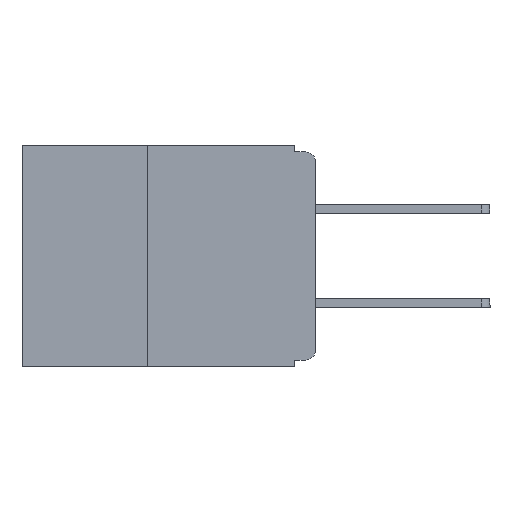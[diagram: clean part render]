
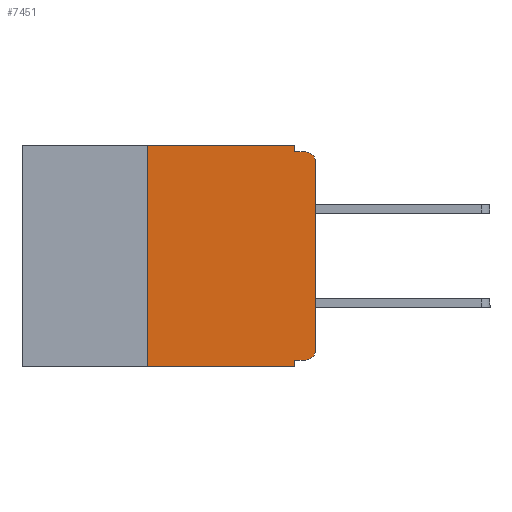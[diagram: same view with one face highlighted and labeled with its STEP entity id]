
A CAD part, left-side view. The second image highlights one B-rep face of the part: STEP entity #7451.
In plain terms, the highlighted planar face has unit normal (-1, 0, 0).
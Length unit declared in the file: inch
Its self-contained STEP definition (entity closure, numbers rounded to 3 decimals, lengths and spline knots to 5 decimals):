
#254 = LINE ( 'NONE', #30132, #18545 ) ;
#297 = CARTESIAN_POINT ( 'NONE',  ( 0., 0.015, -0.01 ) ) ;
#335 = ORIENTED_EDGE ( 'NONE', *, *, #7287, .T. ) ;
#672 = DIRECTION ( 'NONE',  ( 0., -1., 0. ) ) ;
#1065 = VECTOR ( 'NONE', #12411, 39.37008 ) ;
#1700 = CARTESIAN_POINT ( 'NONE',  ( 0., 0., 0. ) ) ;
#1806 = EDGE_LOOP ( 'NONE', ( #30717, #335, #18249, #26218, #25483, #6703, #31536, #11788, #13303, #30813 ) ) ;
#2126 = DIRECTION ( 'NONE',  ( 0., -1., 0. ) ) ;
#2202 = VERTEX_POINT ( 'NONE', #297 ) ;
#2944 = LINE ( 'NONE', #21747, #27592 ) ;
#3209 = CARTESIAN_POINT ( 'NONE',  ( 0., 0.015, -0.305 ) ) ;
#3772 = CARTESIAN_POINT ( 'NONE',  ( 0., 0.25, -0.33 ) ) ;
#4132 = VECTOR ( 'NONE', #2126, 39.37008 ) ;
#4405 = LINE ( 'NONE', #1700, #22552 ) ;
#4862 = DIRECTION ( 'NONE',  ( 0., 0., -1. ) ) ;
#4870 = DIRECTION ( 'NONE',  ( 1., 0., 0. ) ) ;
#4980 = PLANE ( 'NONE',  #14857 ) ;
#5081 = CARTESIAN_POINT ( 'NONE',  ( 0., 0.437, 0. ) ) ;
#5766 = DIRECTION ( 'NONE',  ( 0., 0., -1. ) ) ;
#6234 = VERTEX_POINT ( 'NONE', #24008 ) ;
#6649 = VERTEX_POINT ( 'NONE', #18091 ) ;
#6653 = CARTESIAN_POINT ( 'NONE',  ( 0., 0.25, 0. ) ) ;
#6703 = ORIENTED_EDGE ( 'NONE', *, *, #12889, .F. ) ;
#7101 = CARTESIAN_POINT ( 'NONE',  ( 0., 0.437, 0. ) ) ;
#7257 = VERTEX_POINT ( 'NONE', #7839 ) ;
#7287 = EDGE_CURVE ( 'NONE', #26455, #2202, #21503, .T. ) ;
#7451 = ADVANCED_FACE ( 'NONE', ( #22644 ), #4980, .F. ) ;
#7493 = DIRECTION ( 'NONE',  ( 0., 0., -1. ) ) ;
#7524 = DIRECTION ( 'NONE',  ( -1., 0., 0. ) ) ;
#7559 = CARTESIAN_POINT ( 'NONE',  ( 0., 0.015, -0.025 ) ) ;
#7839 = CARTESIAN_POINT ( 'NONE',  ( 0., 0.015, -0.32 ) ) ;
#10695 = DIRECTION ( 'NONE',  ( 0., -1., 0. ) ) ;
#11396 = CARTESIAN_POINT ( 'NONE',  ( 0., 0.031, 0. ) ) ;
#11788 = ORIENTED_EDGE ( 'NONE', *, *, #17528, .F. ) ;
#11911 = EDGE_CURVE ( 'NONE', #25136, #6649, #254, .T. ) ;
#12411 = DIRECTION ( 'NONE',  ( 0., 0., -1. ) ) ;
#12565 = CIRCLE ( 'NONE', #22914, 0.015 ) ;
#12889 = EDGE_CURVE ( 'NONE', #25136, #25389, #2944, .T. ) ;
#13303 = ORIENTED_EDGE ( 'NONE', *, *, #20411, .F. ) ;
#14413 = VECTOR ( 'NONE', #18692, 39.37008 ) ;
#14503 = VECTOR ( 'NONE', #21837, 39.37008 ) ;
#14857 = AXIS2_PLACEMENT_3D ( 'NONE', #5081, #4870, #4862 ) ;
#16681 = EDGE_CURVE ( 'NONE', #18161, #6234, #21692, .T. ) ;
#17235 = VERTEX_POINT ( 'NONE', #25765 ) ;
#17528 = EDGE_CURVE ( 'NONE', #17235, #6649, #27336, .T. ) ;
#18091 = CARTESIAN_POINT ( 'NONE',  ( 0., 0.031, -0.33 ) ) ;
#18148 = CARTESIAN_POINT ( 'NONE',  ( 0., 0., -0.025 ) ) ;
#18161 = VERTEX_POINT ( 'NONE', #24557 ) ;
#18249 = ORIENTED_EDGE ( 'NONE', *, *, #26424, .F. ) ;
#18545 = VECTOR ( 'NONE', #672, 39.37008 ) ;
#18692 = DIRECTION ( 'NONE',  ( 0., 0., -1. ) ) ;
#20351 = EDGE_CURVE ( 'NONE', #31775, #26455, #4405, .T. ) ;
#20411 = EDGE_CURVE ( 'NONE', #7257, #17235, #21031, .T. ) ;
#20563 = DIRECTION ( 'NONE',  ( -1., 0., 0. ) ) ;
#20694 = EDGE_CURVE ( 'NONE', #7257, #31775, #12565, .T. ) ;
#21031 = LINE ( 'NONE', #29031, #14503 ) ;
#21503 = CIRCLE ( 'NONE', #26906, 0.015 ) ;
#21692 = LINE ( 'NONE', #11396, #14413 ) ;
#21747 = CARTESIAN_POINT ( 'NONE',  ( 0., 0.25, -0.33 ) ) ;
#21837 = DIRECTION ( 'NONE',  ( 0., 1., 0. ) ) ;
#22552 = VECTOR ( 'NONE', #23847, 39.37008 ) ;
#22644 = FACE_OUTER_BOUND ( 'NONE', #1806, .T. ) ;
#22914 = AXIS2_PLACEMENT_3D ( 'NONE', #3209, #20563, #5766 ) ;
#22923 = CARTESIAN_POINT ( 'NONE',  ( 0., 0., -0.01 ) ) ;
#23847 = DIRECTION ( 'NONE',  ( 0., 0., 1. ) ) ;
#24008 = CARTESIAN_POINT ( 'NONE',  ( 0., 0.031, -0.01 ) ) ;
#24183 = DIRECTION ( 'NONE',  ( 0., 0., 1. ) ) ;
#24557 = CARTESIAN_POINT ( 'NONE',  ( 0., 0.031, 0. ) ) ;
#25136 = VERTEX_POINT ( 'NONE', #3772 ) ;
#25389 = VERTEX_POINT ( 'NONE', #6653 ) ;
#25483 = ORIENTED_EDGE ( 'NONE', *, *, #28605, .F. ) ;
#25765 = CARTESIAN_POINT ( 'NONE',  ( 0., 0.031, -0.32 ) ) ;
#26218 = ORIENTED_EDGE ( 'NONE', *, *, #16681, .F. ) ;
#26288 = CARTESIAN_POINT ( 'NONE',  ( 0., 0., -0.305 ) ) ;
#26424 = EDGE_CURVE ( 'NONE', #6234, #2202, #31466, .T. ) ;
#26455 = VERTEX_POINT ( 'NONE', #18148 ) ;
#26906 = AXIS2_PLACEMENT_3D ( 'NONE', #7559, #7524, #7493 ) ;
#27336 = LINE ( 'NONE', #29333, #1065 ) ;
#27592 = VECTOR ( 'NONE', #24183, 39.37008 ) ;
#28605 = EDGE_CURVE ( 'NONE', #25389, #18161, #30979, .T. ) ;
#29031 = CARTESIAN_POINT ( 'NONE',  ( 0., 0., -0.32 ) ) ;
#29333 = CARTESIAN_POINT ( 'NONE',  ( 0., 0.031, -0.33 ) ) ;
#30132 = CARTESIAN_POINT ( 'NONE',  ( 0., 0.437, -0.33 ) ) ;
#30698 = VECTOR ( 'NONE', #10695, 39.37008 ) ;
#30717 = ORIENTED_EDGE ( 'NONE', *, *, #20351, .T. ) ;
#30813 = ORIENTED_EDGE ( 'NONE', *, *, #20694, .T. ) ;
#30979 = LINE ( 'NONE', #7101, #4132 ) ;
#31466 = LINE ( 'NONE', #22923, #30698 ) ;
#31536 = ORIENTED_EDGE ( 'NONE', *, *, #11911, .T. ) ;
#31775 = VERTEX_POINT ( 'NONE', #26288 ) ;
